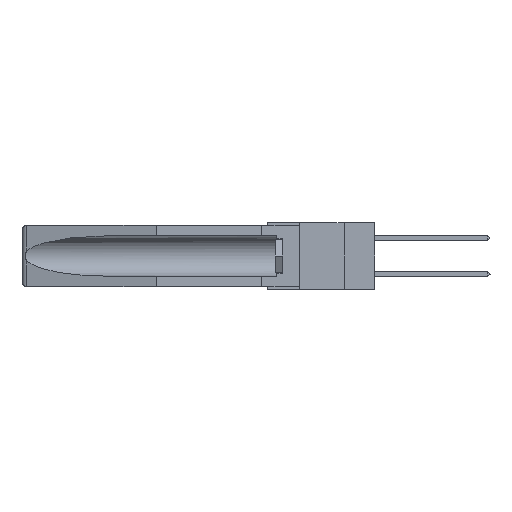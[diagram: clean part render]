
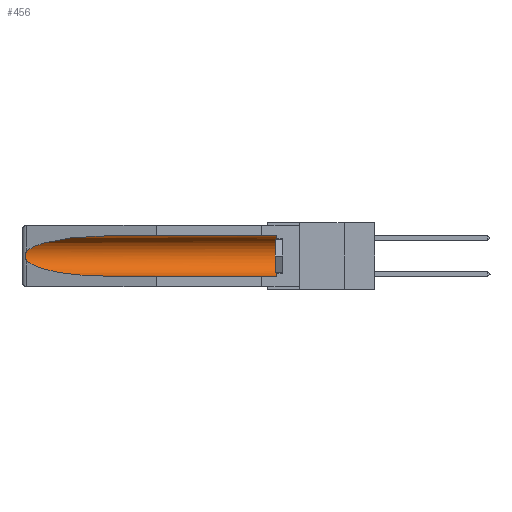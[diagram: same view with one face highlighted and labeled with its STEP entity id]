
A CAD part, left-side view. The second image highlights one B-rep face of the part: STEP entity #456.
In plain terms, the highlighted cylindrical face has radius 2.857 mm (diameter 5.715 mm), a partial arc.
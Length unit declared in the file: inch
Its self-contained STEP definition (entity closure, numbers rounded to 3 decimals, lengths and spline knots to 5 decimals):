
#245 = CARTESIAN_POINT ( 'NONE',  ( 0.155, -0.30754, -0.1715 ) ) ;
#456 = ADVANCED_FACE ( 'NONE', ( #16039 ), #12820, .F. ) ;
#1802 = EDGE_CURVE ( 'NONE', #18729, #7291, #12320, .T. ) ;
#2089 = VERTEX_POINT ( 'NONE', #3389 ) ;
#2216 = CARTESIAN_POINT ( 'NONE',  ( 0.2675, 1.53308, -0.17534 ) ) ;
#2609 = CARTESIAN_POINT ( 'NONE',  ( 0.155, -0.30754, -0.284 ) ) ;
#2696 =( BOUNDED_CURVE ( )  B_SPLINE_CURVE ( 3, ( #11087, #9724, #8102, #12747 ),
 .UNSPECIFIED., .F., .T. ) 
 B_SPLINE_CURVE_WITH_KNOTS ( ( 4, 4 ),
 ( 4.71239, 6.08839 ),
 .UNSPECIFIED. ) 
 CURVE ( )  GEOMETRIC_REPRESENTATION_ITEM ( )  RATIONAL_B_SPLINE_CURVE ( ( 1., 0.848, 0.848, 1. ) ) 
 REPRESENTATION_ITEM ( '' )  );
#2886 = EDGE_CURVE ( 'NONE', #7291, #7320, #2696, .T. ) ;
#3389 = CARTESIAN_POINT ( 'NONE',  ( 0.155, 1.07973, -0.284 ) ) ;
#4036 = CARTESIAN_POINT ( 'NONE',  ( 0.21114, 1.30732, -0.284 ) ) ;
#4623 = CARTESIAN_POINT ( 'NONE',  ( 0.2675, 1.53308, -0.16763 ) ) ;
#4810 = AXIS2_PLACEMENT_3D ( 'NONE', #8118, #10978, #12449 ) ;
#6109 = DIRECTION ( 'NONE',  ( 0., 0., 1. ) ) ;
#6615 = EDGE_CURVE ( 'NONE', #17874, #2089, #15104, .T. ) ;
#6824 = CARTESIAN_POINT ( 'NONE',  ( 0.26597, 1.5296, -0.19026 ) ) ;
#6939 = CARTESIAN_POINT ( 'NONE',  ( 0.26654, 1.53092, -0.15636 ) ) ;
#7102 = ORIENTED_EDGE ( 'NONE', *, *, #7959, .T. ) ;
#7178 = CARTESIAN_POINT ( 'NONE',  ( 0.26537, 1.52718, -0.19328 ) ) ;
#7291 = VERTEX_POINT ( 'NONE', #9162 ) ;
#7312 = CARTESIAN_POINT ( 'NONE',  ( 0.155, -0.30754, -0.059 ) ) ;
#7320 = VERTEX_POINT ( 'NONE', #7912 ) ;
#7912 = CARTESIAN_POINT ( 'NONE',  ( 0.26537, 1.52718, -0.14972 ) ) ;
#7959 = EDGE_CURVE ( 'NONE', #7320, #17874, #11466, .T. ) ;
#8102 = CARTESIAN_POINT ( 'NONE',  ( 0.25451, 1.48313, -0.09465 ) ) ;
#8118 = CARTESIAN_POINT ( 'NONE',  ( 0.155, 0.126, -0.1715 ) ) ;
#8190 = VECTOR ( 'NONE', #16146, 39.37008 ) ;
#8388 = CARTESIAN_POINT ( 'NONE',  ( 0.155, 1.07973, -0.284 ) ) ;
#8595 = CARTESIAN_POINT ( 'NONE',  ( 0.155, 0.126, -0.059 ) ) ;
#9162 = CARTESIAN_POINT ( 'NONE',  ( 0.155, 1.07973, -0.059 ) ) ;
#9724 = CARTESIAN_POINT ( 'NONE',  ( 0.21114, 1.30732, -0.059 ) ) ;
#9774 = ORIENTED_EDGE ( 'NONE', *, *, #13613, .F. ) ;
#10978 = DIRECTION ( 'NONE',  ( 0., -1., 0. ) ) ;
#11087 = CARTESIAN_POINT ( 'NONE',  ( 0.155, 1.07973, -0.059 ) ) ;
#11215 = DIRECTION ( 'NONE',  ( 0., 1., 0. ) ) ;
#11314 = EDGE_LOOP ( 'NONE', ( #16275, #7102, #13487, #9774, #13013, #13968 ) ) ;
#11382 = CARTESIAN_POINT ( 'NONE',  ( 0.25451, 1.48313, -0.24835 ) ) ;
#11466 = B_SPLINE_CURVE_WITH_KNOTS ( 'NONE', 3,
 ( #13533, #11791, #6939, #17203, #4623, #2216, #14117, #16400, #6824, #18621 ),
 .UNSPECIFIED., .F., .F.,
 ( 4, 2, 2, 2, 4 ),
 ( 0., 0.00029, 0.00058, 0.00087, 0.00117 ),
 .UNSPECIFIED. ) ;
#11791 = CARTESIAN_POINT ( 'NONE',  ( 0.26597, 1.52961, -0.15275 ) ) ;
#12232 = VECTOR ( 'NONE', #11215, 39.37008 ) ;
#12320 = LINE ( 'NONE', #7312, #8190 ) ;
#12449 = DIRECTION ( 'NONE',  ( 0., 0., 1. ) ) ;
#12747 = CARTESIAN_POINT ( 'NONE',  ( 0.26537, 1.52718, -0.14972 ) ) ;
#12820 = CYLINDRICAL_SURFACE ( 'NONE', #14855, 0.1125 ) ;
#13013 = ORIENTED_EDGE ( 'NONE', *, *, #14734, .T. ) ;
#13487 = ORIENTED_EDGE ( 'NONE', *, *, #6615, .T. ) ;
#13533 = CARTESIAN_POINT ( 'NONE',  ( 0.26537, 1.52718, -0.14972 ) ) ;
#13613 = EDGE_CURVE ( 'NONE', #17765, #2089, #16143, .T. ) ;
#13968 = ORIENTED_EDGE ( 'NONE', *, *, #1802, .T. ) ;
#14117 = CARTESIAN_POINT ( 'NONE',  ( 0.2673, 1.53269, -0.17917 ) ) ;
#14734 = EDGE_CURVE ( 'NONE', #17765, #18729, #15614, .T. ) ;
#14855 = AXIS2_PLACEMENT_3D ( 'NONE', #245, #14857, #6109 ) ;
#14857 = DIRECTION ( 'NONE',  ( 0., 1., 0. ) ) ;
#15076 = CARTESIAN_POINT ( 'NONE',  ( 0.155, 0.126, -0.284 ) ) ;
#15104 =( BOUNDED_CURVE ( )  B_SPLINE_CURVE ( 3, ( #7178, #11382, #4036, #8388 ),
 .UNSPECIFIED., .F., .F. ) 
 B_SPLINE_CURVE_WITH_KNOTS ( ( 4, 4 ),
 ( 0.1948, 1.5708 ),
 .UNSPECIFIED. ) 
 CURVE ( )  GEOMETRIC_REPRESENTATION_ITEM ( )  RATIONAL_B_SPLINE_CURVE ( ( 1., 0.848, 0.848, 1. ) ) 
 REPRESENTATION_ITEM ( '' )  );
#15614 = CIRCLE ( 'NONE', #4810, 0.1125 ) ;
#16039 = FACE_OUTER_BOUND ( 'NONE', #11314, .T. ) ;
#16143 = LINE ( 'NONE', #2609, #12232 ) ;
#16146 = DIRECTION ( 'NONE',  ( 0., 1., 0. ) ) ;
#16275 = ORIENTED_EDGE ( 'NONE', *, *, #2886, .T. ) ;
#16400 = CARTESIAN_POINT ( 'NONE',  ( 0.26655, 1.53094, -0.18657 ) ) ;
#17203 = CARTESIAN_POINT ( 'NONE',  ( 0.2673, 1.5327, -0.16383 ) ) ;
#17765 = VERTEX_POINT ( 'NONE', #15076 ) ;
#17874 = VERTEX_POINT ( 'NONE', #18807 ) ;
#18621 = CARTESIAN_POINT ( 'NONE',  ( 0.26537, 1.52718, -0.19328 ) ) ;
#18729 = VERTEX_POINT ( 'NONE', #8595 ) ;
#18807 = CARTESIAN_POINT ( 'NONE',  ( 0.26537, 1.52718, -0.19328 ) ) ;
